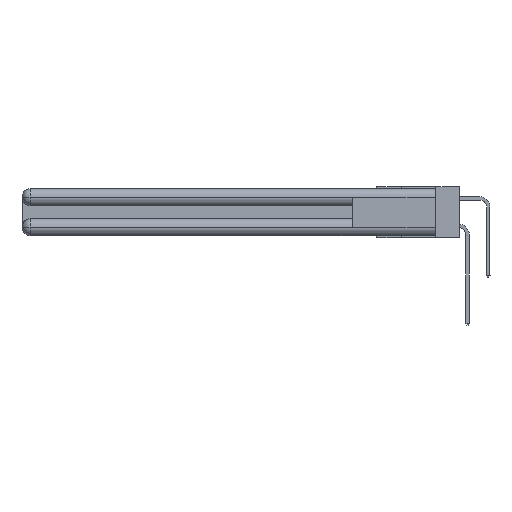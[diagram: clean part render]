
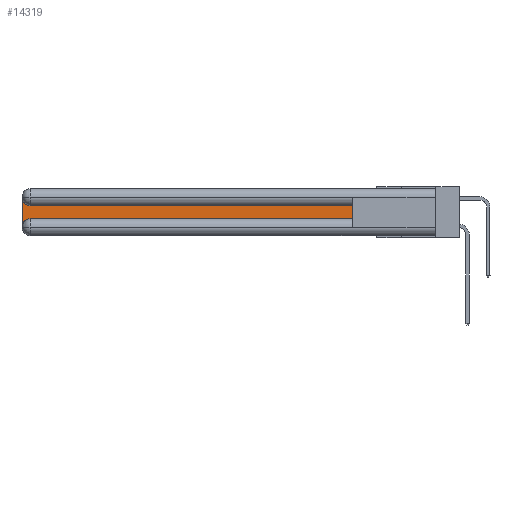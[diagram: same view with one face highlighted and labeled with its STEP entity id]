
A CAD part, left-side view. The second image highlights one B-rep face of the part: STEP entity #14319.
In plain terms, the highlighted planar face has unit normal (-1, 0, 0).
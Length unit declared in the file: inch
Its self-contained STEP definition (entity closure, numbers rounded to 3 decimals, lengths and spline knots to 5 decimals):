
#403 = DIRECTION ( 'NONE',  ( 0., 0., -1. ) ) ;
#1705 = VERTEX_POINT ( 'NONE', #4415 ) ;
#2259 = CIRCLE ( 'NONE', #8603, 0.06 ) ;
#2305 = ORIENTED_EDGE ( 'NONE', *, *, #28399, .T. ) ;
#2491 = VECTOR ( 'NONE', #15356, 39.37008 ) ;
#3302 = EDGE_CURVE ( 'NONE', #13085, #3411, #5040, .T. ) ;
#3411 = VERTEX_POINT ( 'NONE', #18942 ) ;
#4051 = PLANE ( 'NONE',  #5967 ) ;
#4415 = CARTESIAN_POINT ( 'NONE',  ( 0.075, 0.6, -0.2175 ) ) ;
#5040 = LINE ( 'NONE', #20917, #26959 ) ;
#5381 = FACE_OUTER_BOUND ( 'NONE', #13388, .T. ) ;
#5788 = EDGE_CURVE ( 'NONE', #28284, #25161, #2259, .T. ) ;
#5798 = LINE ( 'NONE', #10486, #2491 ) ;
#5967 = AXIS2_PLACEMENT_3D ( 'NONE', #25624, #23422, #18664 ) ;
#8313 = AXIS2_PLACEMENT_3D ( 'NONE', #16074, #25407, #30086 ) ;
#8603 = AXIS2_PLACEMENT_3D ( 'NONE', #16530, #21603, #9673 ) ;
#9673 = DIRECTION ( 'NONE',  ( 0., 0., -1. ) ) ;
#10486 = CARTESIAN_POINT ( 'NONE',  ( 0.075, 0.6, -0.2175 ) ) ;
#10525 = VECTOR ( 'NONE', #403, 39.37008 ) ;
#10976 = CARTESIAN_POINT ( 'NONE',  ( 0.075, 2.94, -0.2175 ) ) ;
#11621 = CARTESIAN_POINT ( 'NONE',  ( 0.075, 3., -0.0625 ) ) ;
#13085 = VERTEX_POINT ( 'NONE', #23845 ) ;
#13388 = EDGE_LOOP ( 'NONE', ( #14608, #2305, #21044, #21690, #22991, #21621 ) ) ;
#13624 = EDGE_CURVE ( 'NONE', #1705, #13085, #5798, .T. ) ;
#13634 = DIRECTION ( 'NONE',  ( 0., 1., 0. ) ) ;
#14319 = ADVANCED_FACE ( 'NONE', ( #5381 ), #4051, .F. ) ;
#14608 = ORIENTED_EDGE ( 'NONE', *, *, #3302, .T. ) ;
#15021 = EDGE_CURVE ( 'NONE', #23615, #28284, #19807, .T. ) ;
#15356 = DIRECTION ( 'NONE',  ( 0., 0., 1. ) ) ;
#15358 = LINE ( 'NONE', #22594, #18367 ) ;
#16074 = CARTESIAN_POINT ( 'NONE',  ( 0.075, 2.94, -0.0625 ) ) ;
#16530 = CARTESIAN_POINT ( 'NONE',  ( 0.075, 2.94, -0.2775 ) ) ;
#18367 = VECTOR ( 'NONE', #20002, 39.37008 ) ;
#18664 = DIRECTION ( 'NONE',  ( 0., 0., -1. ) ) ;
#18942 = CARTESIAN_POINT ( 'NONE',  ( 0.075, 2.94, -0.1225 ) ) ;
#19807 = LINE ( 'NONE', #24264, #10525 ) ;
#20002 = DIRECTION ( 'NONE',  ( 0., -1., 0. ) ) ;
#20917 = CARTESIAN_POINT ( 'NONE',  ( 0.075, 0.6, -0.1225 ) ) ;
#21044 = ORIENTED_EDGE ( 'NONE', *, *, #15021, .T. ) ;
#21603 = DIRECTION ( 'NONE',  ( 1., 0., 0. ) ) ;
#21621 = ORIENTED_EDGE ( 'NONE', *, *, #13624, .T. ) ;
#21690 = ORIENTED_EDGE ( 'NONE', *, *, #5788, .T. ) ;
#22594 = CARTESIAN_POINT ( 'NONE',  ( 0.075, 0.6, -0.2175 ) ) ;
#22686 = CARTESIAN_POINT ( 'NONE',  ( 0.075, 3., -0.2775 ) ) ;
#22991 = ORIENTED_EDGE ( 'NONE', *, *, #30457, .T. ) ;
#23422 = DIRECTION ( 'NONE',  ( 1., 0., 0. ) ) ;
#23615 = VERTEX_POINT ( 'NONE', #11621 ) ;
#23845 = CARTESIAN_POINT ( 'NONE',  ( 0.075, 0.6, -0.1225 ) ) ;
#24264 = CARTESIAN_POINT ( 'NONE',  ( 0.075, 3., -0.2175 ) ) ;
#25161 = VERTEX_POINT ( 'NONE', #10976 ) ;
#25407 = DIRECTION ( 'NONE',  ( 1., 0., 0. ) ) ;
#25624 = CARTESIAN_POINT ( 'NONE',  ( 0.075, 3., -0.1225 ) ) ;
#26522 = CIRCLE ( 'NONE', #8313, 0.06 ) ;
#26959 = VECTOR ( 'NONE', #13634, 39.37008 ) ;
#28284 = VERTEX_POINT ( 'NONE', #22686 ) ;
#28399 = EDGE_CURVE ( 'NONE', #3411, #23615, #26522, .T. ) ;
#30086 = DIRECTION ( 'NONE',  ( 0., 0., -1. ) ) ;
#30457 = EDGE_CURVE ( 'NONE', #25161, #1705, #15358, .T. ) ;
